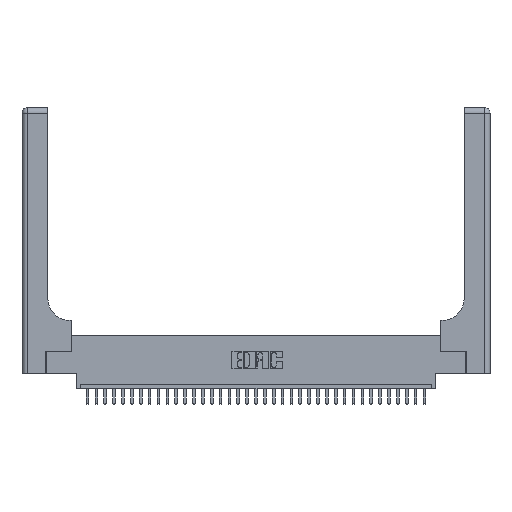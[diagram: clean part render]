
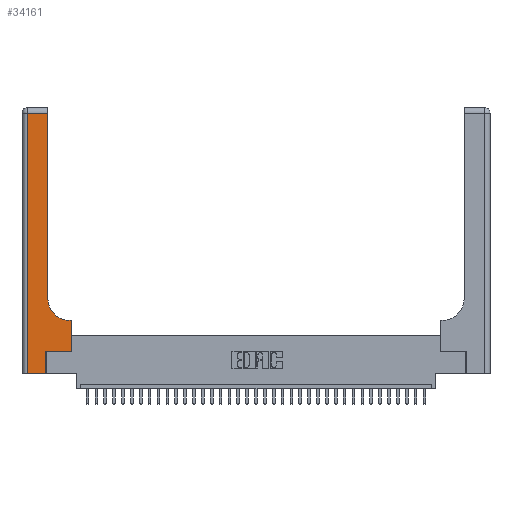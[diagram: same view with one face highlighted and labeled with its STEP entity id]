
A CAD part, top view. The second image highlights one B-rep face of the part: STEP entity #34161.
In plain terms, the highlighted planar face has unit normal (0, 0, 1).
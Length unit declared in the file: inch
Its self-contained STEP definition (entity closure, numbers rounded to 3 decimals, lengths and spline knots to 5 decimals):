
#93 = VERTEX_POINT ( 'NONE', #22774 ) ;
#975 = EDGE_LOOP ( 'NONE', ( #33807, #19999, #28677, #21181, #1120, #12752, #23215, #16533, #34377 ) ) ;
#1120 = ORIENTED_EDGE ( 'NONE', *, *, #19958, .T. ) ;
#1494 = AXIS2_PLACEMENT_3D ( 'NONE', #9478, #22789, #23026 ) ;
#1625 = VERTEX_POINT ( 'NONE', #25821 ) ;
#2130 = DIRECTION ( 'NONE',  ( 1., 0., 0. ) ) ;
#2729 = EDGE_CURVE ( 'NONE', #15050, #1625, #16545, .T. ) ;
#3862 = DIRECTION ( 'NONE',  ( -1., 0., 0. ) ) ;
#5241 = VECTOR ( 'NONE', #15868, 39.37008 ) ;
#6410 = PLANE ( 'NONE',  #26360 ) ;
#7714 = LINE ( 'NONE', #18139, #13674 ) ;
#8008 = CARTESIAN_POINT ( 'NONE',  ( 0.269, 0., 0.37 ) ) ;
#9478 = CARTESIAN_POINT ( 'NONE',  ( 0.5415, 0.85, 0.37 ) ) ;
#10028 = VECTOR ( 'NONE', #19908, 39.37008 ) ;
#10347 = VECTOR ( 'NONE', #29351, 39.37008 ) ;
#10597 = CARTESIAN_POINT ( 'NONE',  ( 0.5585, 0.6, 0.37 ) ) ;
#10978 = EDGE_CURVE ( 'NONE', #93, #29718, #19226, .T. ) ;
#12583 = LINE ( 'NONE', #14437, #10028 ) ;
#12752 = ORIENTED_EDGE ( 'NONE', *, *, #22354, .T. ) ;
#12770 = VECTOR ( 'NONE', #33937, 39.37008 ) ;
#12940 = CARTESIAN_POINT ( 'NONE',  ( 0., 2.94, 0.37 ) ) ;
#13104 = LINE ( 'NONE', #34070, #29213 ) ;
#13374 = VERTEX_POINT ( 'NONE', #32692 ) ;
#13674 = VECTOR ( 'NONE', #2130, 39.37008 ) ;
#13916 = LINE ( 'NONE', #15828, #22853 ) ;
#14137 = DIRECTION ( 'NONE',  ( -1., 0., 0. ) ) ;
#14437 = CARTESIAN_POINT ( 'NONE',  ( 0.5585, 0.25, 0.37 ) ) ;
#14462 = LINE ( 'NONE', #34298, #12770 ) ;
#15050 = VERTEX_POINT ( 'NONE', #23831 ) ;
#15828 = CARTESIAN_POINT ( 'NONE',  ( 0.06, 3., 0.37 ) ) ;
#15868 = DIRECTION ( 'NONE',  ( 0., 1., 0. ) ) ;
#16418 = EDGE_CURVE ( 'NONE', #29718, #13374, #13916, .T. ) ;
#16533 = ORIENTED_EDGE ( 'NONE', *, *, #21882, .T. ) ;
#16545 = CIRCLE ( 'NONE', #1494, 0.25 ) ;
#16735 = CARTESIAN_POINT ( 'NONE',  ( 0., 3., 0.37 ) ) ;
#18139 = CARTESIAN_POINT ( 'NONE',  ( 0., 0., 0.37 ) ) ;
#19226 = LINE ( 'NONE', #12940, #10347 ) ;
#19558 = CARTESIAN_POINT ( 'NONE',  ( 0.269, 0.25, 0.37 ) ) ;
#19657 = LINE ( 'NONE', #8008, #5241 ) ;
#19908 = DIRECTION ( 'NONE',  ( 0., 1., 0. ) ) ;
#19958 = EDGE_CURVE ( 'NONE', #22651, #30084, #19657, .T. ) ;
#19999 = ORIENTED_EDGE ( 'NONE', *, *, #10978, .T. ) ;
#20863 = EDGE_CURVE ( 'NONE', #13374, #22651, #7714, .T. ) ;
#21181 = ORIENTED_EDGE ( 'NONE', *, *, #20863, .T. ) ;
#21882 = EDGE_CURVE ( 'NONE', #25883, #15050, #13104, .T. ) ;
#22354 = EDGE_CURVE ( 'NONE', #30084, #24570, #33037, .T. ) ;
#22651 = VERTEX_POINT ( 'NONE', #26222 ) ;
#22774 = CARTESIAN_POINT ( 'NONE',  ( 0.2915, 2.94, 0.37 ) ) ;
#22789 = DIRECTION ( 'NONE',  ( 0., 0., -1. ) ) ;
#22796 = DIRECTION ( 'NONE',  ( 1., 0., 0. ) ) ;
#22853 = VECTOR ( 'NONE', #30252, 39.37008 ) ;
#23026 = DIRECTION ( 'NONE',  ( 1., 0., 0. ) ) ;
#23162 = EDGE_CURVE ( 'NONE', #24570, #25883, #12583, .T. ) ;
#23215 = ORIENTED_EDGE ( 'NONE', *, *, #23162, .T. ) ;
#23831 = CARTESIAN_POINT ( 'NONE',  ( 0.5415, 0.6, 0.37 ) ) ;
#24570 = VERTEX_POINT ( 'NONE', #35088 ) ;
#24821 = FACE_OUTER_BOUND ( 'NONE', #975, .T. ) ;
#24947 = DIRECTION ( 'NONE',  ( 0., 0., -1. ) ) ;
#25821 = CARTESIAN_POINT ( 'NONE',  ( 0.2915, 0.85, 0.37 ) ) ;
#25883 = VERTEX_POINT ( 'NONE', #10597 ) ;
#26222 = CARTESIAN_POINT ( 'NONE',  ( 0.269, 0., 0.37 ) ) ;
#26360 = AXIS2_PLACEMENT_3D ( 'NONE', #16735, #24947, #14137 ) ;
#26655 = VECTOR ( 'NONE', #22796, 39.37008 ) ;
#28677 = ORIENTED_EDGE ( 'NONE', *, *, #16418, .T. ) ;
#29213 = VECTOR ( 'NONE', #3862, 39.37008 ) ;
#29351 = DIRECTION ( 'NONE',  ( -1., 0., 0. ) ) ;
#29718 = VERTEX_POINT ( 'NONE', #31165 ) ;
#29750 = EDGE_CURVE ( 'NONE', #1625, #93, #14462, .T. ) ;
#30084 = VERTEX_POINT ( 'NONE', #19558 ) ;
#30252 = DIRECTION ( 'NONE',  ( 0., -1., 0. ) ) ;
#31165 = CARTESIAN_POINT ( 'NONE',  ( 0.06, 2.94, 0.37 ) ) ;
#32692 = CARTESIAN_POINT ( 'NONE',  ( 0.06, 0., 0.37 ) ) ;
#33037 = LINE ( 'NONE', #33569, #26655 ) ;
#33569 = CARTESIAN_POINT ( 'NONE',  ( 0.269, 0.25, 0.37 ) ) ;
#33807 = ORIENTED_EDGE ( 'NONE', *, *, #29750, .T. ) ;
#33937 = DIRECTION ( 'NONE',  ( 0., 1., 0. ) ) ;
#34070 = CARTESIAN_POINT ( 'NONE',  ( 0.2915, 0.6, 0.37 ) ) ;
#34161 = ADVANCED_FACE ( 'NONE', ( #24821 ), #6410, .F. ) ;
#34298 = CARTESIAN_POINT ( 'NONE',  ( 0.2915, 3., 0.37 ) ) ;
#34377 = ORIENTED_EDGE ( 'NONE', *, *, #2729, .T. ) ;
#35088 = CARTESIAN_POINT ( 'NONE',  ( 0.5585, 0.25, 0.37 ) ) ;
